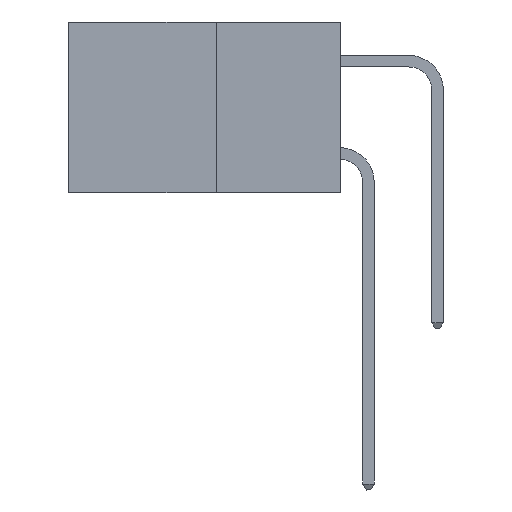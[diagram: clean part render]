
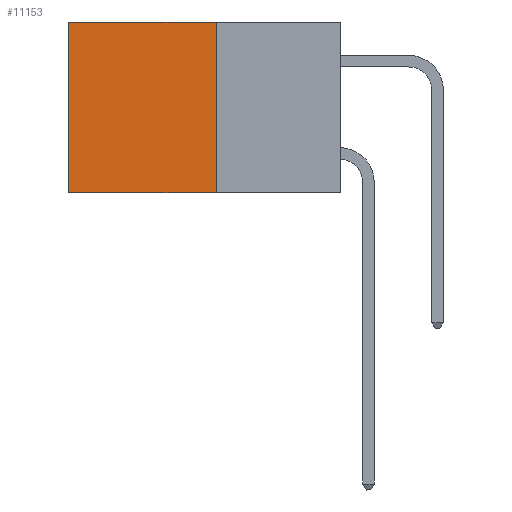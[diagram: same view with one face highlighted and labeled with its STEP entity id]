
A CAD part, left-side view. The second image highlights one B-rep face of the part: STEP entity #11153.
In plain terms, the highlighted planar face has unit normal (-1, 0, 0).
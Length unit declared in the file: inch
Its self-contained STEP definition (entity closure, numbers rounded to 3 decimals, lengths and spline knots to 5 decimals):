
#34 = ORIENTED_EDGE ( 'NONE', *, *, #13613, .F. ) ;
#836 = DIRECTION ( 'NONE',  ( 0., 0., -1. ) ) ;
#2023 = VECTOR ( 'NONE', #11764, 39.37008 ) ;
#2418 = LINE ( 'NONE', #19685, #16916 ) ;
#2979 = AXIS2_PLACEMENT_3D ( 'NONE', #4104, #15526, #4195 ) ;
#3285 = VERTEX_POINT ( 'NONE', #23076 ) ;
#4104 = CARTESIAN_POINT ( 'NONE',  ( 0.277, 0.27, -0.37 ) ) ;
#4195 = DIRECTION ( 'NONE',  ( 0., 0., -1. ) ) ;
#4928 = ORIENTED_EDGE ( 'NONE', *, *, #20941, .F. ) ;
#6010 = ORIENTED_EDGE ( 'NONE', *, *, #20488, .T. ) ;
#6155 = VERTEX_POINT ( 'NONE', #7700 ) ;
#7700 = CARTESIAN_POINT ( 'NONE',  ( 0.277, 0.59, 0. ) ) ;
#8604 = EDGE_CURVE ( 'NONE', #6155, #14285, #2418, .T. ) ;
#8643 = LINE ( 'NONE', #19737, #15725 ) ;
#9832 = CARTESIAN_POINT ( 'NONE',  ( 0.277, 0.27, -0.37 ) ) ;
#9983 = LINE ( 'NONE', #10362, #14410 ) ;
#10339 = CARTESIAN_POINT ( 'NONE',  ( 0.277, 0.59, -0.37 ) ) ;
#10362 = CARTESIAN_POINT ( 'NONE',  ( 0.277, 0.27, -0.37 ) ) ;
#11153 = ADVANCED_FACE ( 'NONE', ( #17074 ), #22704, .F. ) ;
#11580 = LINE ( 'NONE', #9832, #2023 ) ;
#11764 = DIRECTION ( 'NONE',  ( 0., 1., 0. ) ) ;
#12202 = ORIENTED_EDGE ( 'NONE', *, *, #8604, .T. ) ;
#13613 = EDGE_CURVE ( 'NONE', #23905, #3285, #9983, .T. ) ;
#14285 = VERTEX_POINT ( 'NONE', #10339 ) ;
#14410 = VECTOR ( 'NONE', #836, 39.37008 ) ;
#15067 = CARTESIAN_POINT ( 'NONE',  ( 0.277, 0.27, 0. ) ) ;
#15526 = DIRECTION ( 'NONE',  ( 1., 0., 0. ) ) ;
#15725 = VECTOR ( 'NONE', #16160, 39.37008 ) ;
#16160 = DIRECTION ( 'NONE',  ( 0., 1., 0. ) ) ;
#16916 = VECTOR ( 'NONE', #21492, 39.37008 ) ;
#17074 = FACE_OUTER_BOUND ( 'NONE', #20552, .T. ) ;
#19685 = CARTESIAN_POINT ( 'NONE',  ( 0.277, 0.59, -0.37 ) ) ;
#19737 = CARTESIAN_POINT ( 'NONE',  ( 0.277, 0.27, 0. ) ) ;
#20488 = EDGE_CURVE ( 'NONE', #23905, #6155, #8643, .T. ) ;
#20552 = EDGE_LOOP ( 'NONE', ( #12202, #4928, #34, #6010 ) ) ;
#20941 = EDGE_CURVE ( 'NONE', #3285, #14285, #11580, .T. ) ;
#21492 = DIRECTION ( 'NONE',  ( 0., 0., -1. ) ) ;
#22704 = PLANE ( 'NONE',  #2979 ) ;
#23076 = CARTESIAN_POINT ( 'NONE',  ( 0.277, 0.27, -0.37 ) ) ;
#23905 = VERTEX_POINT ( 'NONE', #15067 ) ;
